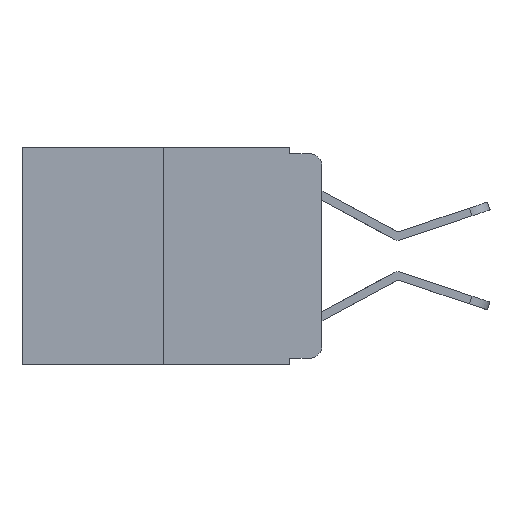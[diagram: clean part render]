
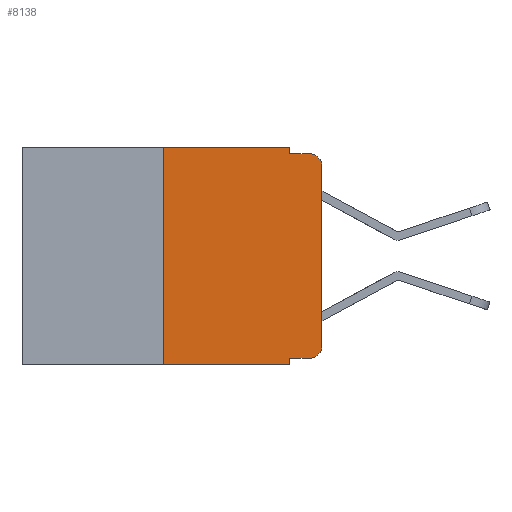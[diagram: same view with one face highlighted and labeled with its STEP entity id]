
A CAD part, left-side view. The second image highlights one B-rep face of the part: STEP entity #8138.
In plain terms, the highlighted planar face has unit normal (-1, 0, 0).
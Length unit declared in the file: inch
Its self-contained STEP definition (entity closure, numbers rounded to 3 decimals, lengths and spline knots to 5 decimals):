
#93 = ORIENTED_EDGE ( 'NONE', *, *, #11546, .F. ) ;
#199 = CARTESIAN_POINT ( 'NONE',  ( 0., 0.02, -0.01 ) ) ;
#236 = VERTEX_POINT ( 'NONE', #7562 ) ;
#489 = EDGE_CURVE ( 'NONE', #15216, #4398, #4309, .T. ) ;
#920 = LINE ( 'NONE', #7761, #2987 ) ;
#1110 = ORIENTED_EDGE ( 'NONE', *, *, #11564, .T. ) ;
#1179 = VERTEX_POINT ( 'NONE', #15278 ) ;
#1271 = DIRECTION ( 'NONE',  ( 0., -1., 0. ) ) ;
#1970 = CARTESIAN_POINT ( 'NONE',  ( 0., 0.02, -0.313 ) ) ;
#2317 = VECTOR ( 'NONE', #15461, 39.37008 ) ;
#2468 = LINE ( 'NONE', #4566, #12258 ) ;
#2987 = VECTOR ( 'NONE', #14430, 39.37008 ) ;
#3378 = VERTEX_POINT ( 'NONE', #9110 ) ;
#3897 = DIRECTION ( 'NONE',  ( 1., 0., 0. ) ) ;
#4309 = LINE ( 'NONE', #14651, #7040 ) ;
#4398 = VERTEX_POINT ( 'NONE', #7353 ) ;
#4566 = CARTESIAN_POINT ( 'NONE',  ( 0., 0.051, 0. ) ) ;
#4583 = VERTEX_POINT ( 'NONE', #10429 ) ;
#4969 = EDGE_CURVE ( 'NONE', #4398, #3378, #2468, .T. ) ;
#5031 = PLANE ( 'NONE',  #16650 ) ;
#5075 = CARTESIAN_POINT ( 'NONE',  ( 0., 0.051, -0.01 ) ) ;
#5213 = FACE_OUTER_BOUND ( 'NONE', #11841, .T. ) ;
#5250 = ORIENTED_EDGE ( 'NONE', *, *, #7540, .T. ) ;
#5352 = EDGE_CURVE ( 'NONE', #1179, #7559, #16834, .T. ) ;
#5632 = ORIENTED_EDGE ( 'NONE', *, *, #12721, .F. ) ;
#5654 = DIRECTION ( 'NONE',  ( -1., 0., 0. ) ) ;
#5830 = DIRECTION ( 'NONE',  ( -1., 0., 0. ) ) ;
#6034 = CARTESIAN_POINT ( 'NONE',  ( 0., 0.25, -0.343 ) ) ;
#6069 = LINE ( 'NONE', #11193, #7126 ) ;
#6476 = DIRECTION ( 'NONE',  ( 0., -1., 0. ) ) ;
#6552 = VERTEX_POINT ( 'NONE', #6034 ) ;
#6571 = LINE ( 'NONE', #5075, #12361 ) ;
#7040 = VECTOR ( 'NONE', #1271, 39.37008 ) ;
#7115 = VECTOR ( 'NONE', #8780, 39.37008 ) ;
#7126 = VECTOR ( 'NONE', #16347, 39.37008 ) ;
#7169 = VERTEX_POINT ( 'NONE', #199 ) ;
#7189 = DIRECTION ( 'NONE',  ( 0., 0., -1. ) ) ;
#7353 = CARTESIAN_POINT ( 'NONE',  ( 0., 0.051, 0. ) ) ;
#7540 = EDGE_CURVE ( 'NONE', #7559, #236, #16029, .T. ) ;
#7559 = VERTEX_POINT ( 'NONE', #12983 ) ;
#7562 = CARTESIAN_POINT ( 'NONE',  ( 0., 0., -0.03 ) ) ;
#7761 = CARTESIAN_POINT ( 'NONE',  ( 0., 0.051, -0.333 ) ) ;
#8138 = ADVANCED_FACE ( 'NONE', ( #5213 ), #5031, .F. ) ;
#8331 = ORIENTED_EDGE ( 'NONE', *, *, #5352, .T. ) ;
#8742 = LINE ( 'NONE', #10224, #14719 ) ;
#8768 = EDGE_CURVE ( 'NONE', #6552, #15216, #8742, .T. ) ;
#8780 = DIRECTION ( 'NONE',  ( 0., 0., 1. ) ) ;
#9110 = CARTESIAN_POINT ( 'NONE',  ( 0., 0.051, -0.01 ) ) ;
#9640 = CARTESIAN_POINT ( 'NONE',  ( 0., 0.051, -0.343 ) ) ;
#9897 = DIRECTION ( 'NONE',  ( 0., 0., -1. ) ) ;
#10224 = CARTESIAN_POINT ( 'NONE',  ( 0., 0.25, 0. ) ) ;
#10429 = CARTESIAN_POINT ( 'NONE',  ( 0., 0.051, -0.333 ) ) ;
#10448 = CARTESIAN_POINT ( 'NONE',  ( 0., 0.25, 0. ) ) ;
#11054 = CARTESIAN_POINT ( 'NONE',  ( 0., 0.02, -0.03 ) ) ;
#11193 = CARTESIAN_POINT ( 'NONE',  ( 0., 0.473, -0.343 ) ) ;
#11435 = ORIENTED_EDGE ( 'NONE', *, *, #15005, .T. ) ;
#11546 = EDGE_CURVE ( 'NONE', #3378, #7169, #6571, .T. ) ;
#11564 = EDGE_CURVE ( 'NONE', #4583, #1179, #920, .T. ) ;
#11841 = EDGE_LOOP ( 'NONE', ( #5250, #16615, #93, #12900, #12788, #14924, #11435, #5632, #1110, #8331 ) ) ;
#12258 = VECTOR ( 'NONE', #9897, 39.37008 ) ;
#12361 = VECTOR ( 'NONE', #6476, 39.37008 ) ;
#12500 = AXIS2_PLACEMENT_3D ( 'NONE', #1970, #5830, #7189 ) ;
#12721 = EDGE_CURVE ( 'NONE', #4583, #15524, #15221, .T. ) ;
#12748 = CIRCLE ( 'NONE', #15734, 0.02 ) ;
#12788 = ORIENTED_EDGE ( 'NONE', *, *, #489, .F. ) ;
#12863 = DIRECTION ( 'NONE',  ( 0., 0., 1. ) ) ;
#12900 = ORIENTED_EDGE ( 'NONE', *, *, #4969, .F. ) ;
#12983 = CARTESIAN_POINT ( 'NONE',  ( 0., 0., -0.313 ) ) ;
#13034 = CARTESIAN_POINT ( 'NONE',  ( 0., 0.473, 0. ) ) ;
#14183 = EDGE_CURVE ( 'NONE', #236, #7169, #12748, .T. ) ;
#14315 = DIRECTION ( 'NONE',  ( 0., 0., -1. ) ) ;
#14430 = DIRECTION ( 'NONE',  ( 0., -1., 0. ) ) ;
#14651 = CARTESIAN_POINT ( 'NONE',  ( 0., 0.473, 0. ) ) ;
#14719 = VECTOR ( 'NONE', #12863, 39.37008 ) ;
#14924 = ORIENTED_EDGE ( 'NONE', *, *, #8768, .F. ) ;
#15005 = EDGE_CURVE ( 'NONE', #6552, #15524, #6069, .T. ) ;
#15216 = VERTEX_POINT ( 'NONE', #10448 ) ;
#15221 = LINE ( 'NONE', #16748, #2317 ) ;
#15278 = CARTESIAN_POINT ( 'NONE',  ( 0., 0.02, -0.333 ) ) ;
#15461 = DIRECTION ( 'NONE',  ( 0., 0., -1. ) ) ;
#15524 = VERTEX_POINT ( 'NONE', #9640 ) ;
#15734 = AXIS2_PLACEMENT_3D ( 'NONE', #11054, #5654, #16368 ) ;
#16029 = LINE ( 'NONE', #16646, #7115 ) ;
#16347 = DIRECTION ( 'NONE',  ( 0., -1., 0. ) ) ;
#16368 = DIRECTION ( 'NONE',  ( 0., 0., -1. ) ) ;
#16615 = ORIENTED_EDGE ( 'NONE', *, *, #14183, .T. ) ;
#16646 = CARTESIAN_POINT ( 'NONE',  ( 0., 0., 0. ) ) ;
#16650 = AXIS2_PLACEMENT_3D ( 'NONE', #13034, #3897, #14315 ) ;
#16748 = CARTESIAN_POINT ( 'NONE',  ( 0., 0.051, 0. ) ) ;
#16834 = CIRCLE ( 'NONE', #12500, 0.02 ) ;
